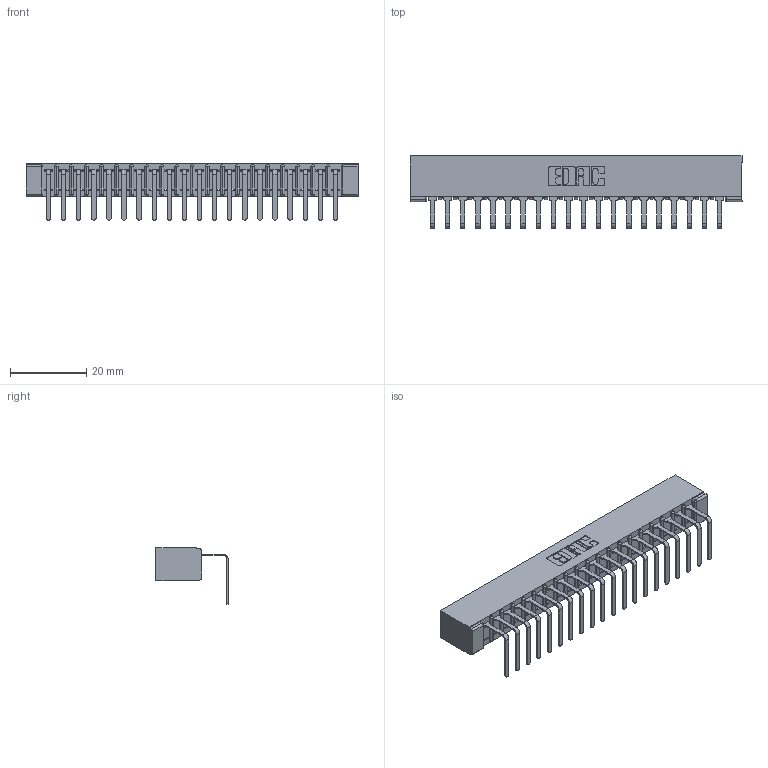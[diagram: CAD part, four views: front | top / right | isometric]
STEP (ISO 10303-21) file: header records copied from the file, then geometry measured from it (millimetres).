
FILE_DESCRIPTION (( 'STEP AP203' ), '1' );
FILE_NAME ('307-020-558-101.STEP', '2019-09-04T13:13:55', ( '' ), ( '' ), 'SwSTEP 2.0', 'SolidWorks 2016', '' );
FILE_SCHEMA (( 'CONFIG_CONTROL_DESIGN' ));
Length unit declared in the file: inch
Products named in the file (3): 307-290-001_558 - 2 (Single); 307 Part_No Mounting Lugs; 307-020-558-101
Assembly tree (21 placements, depth 2):
  307-020-558-101
    307 Part_No Mounting Lugs
    307-290-001_558 - 2 (Single)  x20
Bounding box: 87.12 x 18.96 x 14.81 mm (x, y, z)
Volume: 5794.9 mm3; surface area: 9770.3 mm2
Topology: 21 solids, 21 shells, 1331 faces, 3779 edges, 2434 vertices
Faces by surface type: plane 846, cylinder 443, sphere 42
Entity records: 19684 total; most frequent: CARTESIAN_POINT 3308, ORIENTED_EDGE 3294, DIRECTION 3229, EDGE_CURVE 1647, LINE 1255, VECTOR 1255, VERTEX_POINT 1066, AXIS2_PLACEMENT_3D 987
